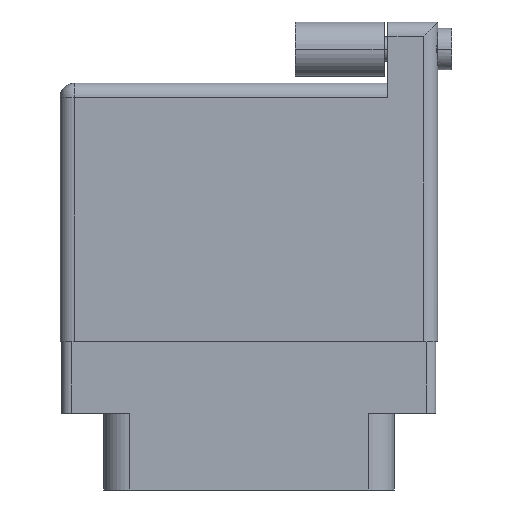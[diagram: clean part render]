
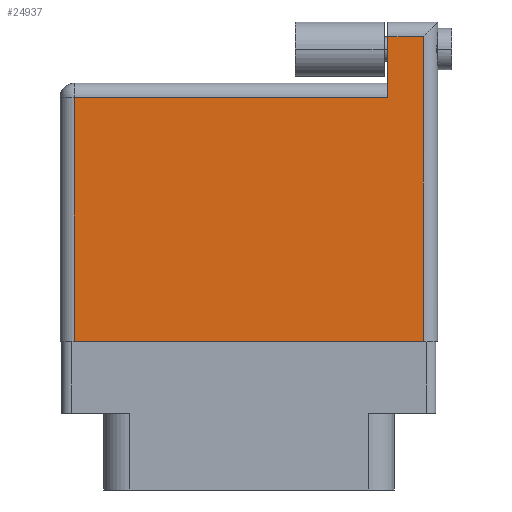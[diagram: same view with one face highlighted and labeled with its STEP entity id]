
A CAD part, front view. The second image highlights one B-rep face of the part: STEP entity #24937.
In plain terms, the highlighted face is planar.
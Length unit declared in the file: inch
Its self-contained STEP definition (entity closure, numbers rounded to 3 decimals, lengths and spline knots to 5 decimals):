
#33 = ORIENTED_EDGE ( 'NONE', *, *, #5633, .T. ) ;
#1291 = VECTOR ( 'NONE', #11595, 39.37008 ) ;
#2964 = LINE ( 'NONE', #21385, #17942 ) ;
#3739 = CARTESIAN_POINT ( 'NONE',  ( 1.275, 0., 0. ) ) ;
#3959 = CARTESIAN_POINT ( 'NONE',  ( 0.05, 0.856, 0. ) ) ;
#5063 = LINE ( 'NONE', #7637, #14010 ) ;
#5633 = EDGE_CURVE ( 'NONE', #16752, #14965, #20135, .T. ) ;
#7101 = VECTOR ( 'NONE', #22483, 39.37008 ) ;
#7316 = LINE ( 'NONE', #7455, #1291 ) ;
#7455 = CARTESIAN_POINT ( 'NONE',  ( 0.05, 0., 0. ) ) ;
#7637 = CARTESIAN_POINT ( 'NONE',  ( 0., 1.07, 0. ) ) ;
#7660 = EDGE_CURVE ( 'NONE', #25603, #12179, #17965, .T. ) ;
#7943 = EDGE_CURVE ( 'NONE', #12179, #21104, #2964, .T. ) ;
#8134 = DIRECTION ( 'NONE',  ( 0., 1., 0. ) ) ;
#9225 = DIRECTION ( 'NONE',  ( 0., 0., -1. ) ) ;
#9406 = DIRECTION ( 'NONE',  ( -1., 0., 0. ) ) ;
#10053 = DIRECTION ( 'NONE',  ( 1., 0., 0. ) ) ;
#10380 = CARTESIAN_POINT ( 'NONE',  ( 1.15, 0.856, 0. ) ) ;
#11595 = DIRECTION ( 'NONE',  ( 0., -1., 0. ) ) ;
#11751 = VECTOR ( 'NONE', #8134, 39.37008 ) ;
#12008 = EDGE_CURVE ( 'NONE', #14965, #25862, #23232, .T. ) ;
#12111 = CARTESIAN_POINT ( 'NONE',  ( 0.05, 0., 0. ) ) ;
#12179 = VERTEX_POINT ( 'NONE', #10380 ) ;
#12350 = ORIENTED_EDGE ( 'NONE', *, *, #12008, .T. ) ;
#13199 = ORIENTED_EDGE ( 'NONE', *, *, #18377, .T. ) ;
#13588 = ORIENTED_EDGE ( 'NONE', *, *, #7660, .T. ) ;
#13668 = CARTESIAN_POINT ( 'NONE',  ( 1.15, 1.07, 0. ) ) ;
#13925 = AXIS2_PLACEMENT_3D ( 'NONE', #19756, #9225, #9406 ) ;
#14010 = VECTOR ( 'NONE', #21860, 39.37008 ) ;
#14066 = VECTOR ( 'NONE', #10053, 39.37008 ) ;
#14965 = VERTEX_POINT ( 'NONE', #3739 ) ;
#16278 = CARTESIAN_POINT ( 'NONE',  ( 0., 0., 0. ) ) ;
#16488 = CARTESIAN_POINT ( 'NONE',  ( 1.275, 1.07, 0. ) ) ;
#16752 = VERTEX_POINT ( 'NONE', #12111 ) ;
#16875 = FACE_OUTER_BOUND ( 'NONE', #18402, .T. ) ;
#17521 = PLANE ( 'NONE',  #13925 ) ;
#17942 = VECTOR ( 'NONE', #23437, 39.37008 ) ;
#17965 = LINE ( 'NONE', #20253, #7101 ) ;
#18377 = EDGE_CURVE ( 'NONE', #25862, #25603, #5063, .T. ) ;
#18402 = EDGE_LOOP ( 'NONE', ( #33, #12350, #13199, #13588, #25510, #25407 ) ) ;
#19756 = CARTESIAN_POINT ( 'NONE',  ( 0., 0.906, 0. ) ) ;
#20135 = LINE ( 'NONE', #16278, #14066 ) ;
#20253 = CARTESIAN_POINT ( 'NONE',  ( 1.15, 1.12, 0. ) ) ;
#21104 = VERTEX_POINT ( 'NONE', #3959 ) ;
#21385 = CARTESIAN_POINT ( 'NONE',  ( 0., 0.856, 0. ) ) ;
#21860 = DIRECTION ( 'NONE',  ( -1., 0., 0. ) ) ;
#22260 = CARTESIAN_POINT ( 'NONE',  ( 1.275, 1.12, 0. ) ) ;
#22483 = DIRECTION ( 'NONE',  ( 0., -1., 0. ) ) ;
#23232 = LINE ( 'NONE', #22260, #11751 ) ;
#23437 = DIRECTION ( 'NONE',  ( -1., 0., 0. ) ) ;
#24564 = EDGE_CURVE ( 'NONE', #21104, #16752, #7316, .T. ) ;
#24937 = ADVANCED_FACE ( 'NONE', ( #16875 ), #17521, .F. ) ;
#25407 = ORIENTED_EDGE ( 'NONE', *, *, #24564, .T. ) ;
#25510 = ORIENTED_EDGE ( 'NONE', *, *, #7943, .T. ) ;
#25603 = VERTEX_POINT ( 'NONE', #13668 ) ;
#25862 = VERTEX_POINT ( 'NONE', #16488 ) ;
